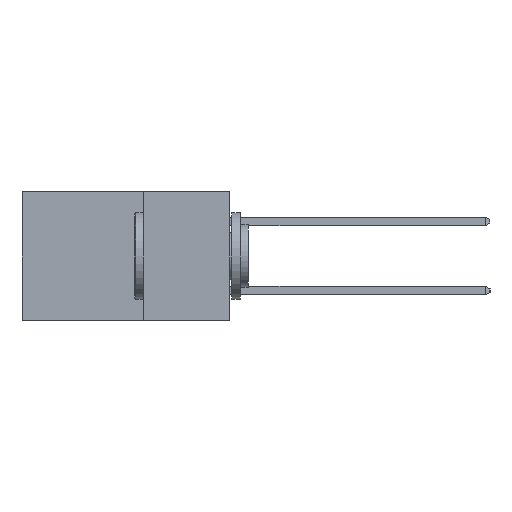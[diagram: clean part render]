
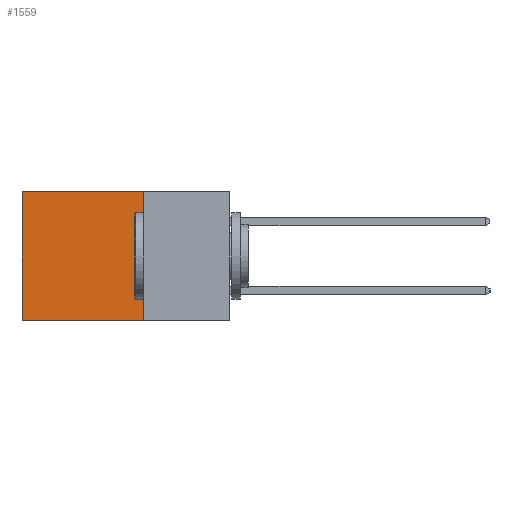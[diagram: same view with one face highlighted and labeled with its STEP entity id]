
A CAD part, left-side view. The second image highlights one B-rep face of the part: STEP entity #1559.
In plain terms, the highlighted planar face has unit normal (-1, 0, 0).
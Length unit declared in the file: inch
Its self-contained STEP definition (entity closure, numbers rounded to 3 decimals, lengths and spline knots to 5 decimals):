
#1008 = AXIS2_PLACEMENT_3D ( 'NONE', #8813, #7997, #16315 ) ;
#1194 = ORIENTED_EDGE ( 'NONE', *, *, #7475, .F. ) ;
#1559 = ADVANCED_FACE ( 'NONE', ( #24263 ), #5330, .F. ) ;
#2029 = CARTESIAN_POINT ( 'NONE',  ( 0.2615, 0.25, -0.37 ) ) ;
#2260 = ORIENTED_EDGE ( 'NONE', *, *, #23071, .T. ) ;
#2371 = VECTOR ( 'NONE', #18679, 39.37008 ) ;
#4174 = DIRECTION ( 'NONE',  ( 0., 0., -1. ) ) ;
#5225 = VERTEX_POINT ( 'NONE', #13977 ) ;
#5330 = PLANE ( 'NONE',  #1008 ) ;
#5928 = EDGE_CURVE ( 'NONE', #17173, #8395, #12949, .T. ) ;
#6491 = ORIENTED_EDGE ( 'NONE', *, *, #5928, .F. ) ;
#7475 = EDGE_CURVE ( 'NONE', #8395, #22567, #9913, .T. ) ;
#7939 = VECTOR ( 'NONE', #23705, 39.37008 ) ;
#7997 = DIRECTION ( 'NONE',  ( 1., 0., 0. ) ) ;
#8395 = VERTEX_POINT ( 'NONE', #2029 ) ;
#8813 = CARTESIAN_POINT ( 'NONE',  ( 0.2615, 0.25, -0.37 ) ) ;
#9248 = CARTESIAN_POINT ( 'NONE',  ( 0.2615, 0.25, 0. ) ) ;
#9913 = LINE ( 'NONE', #11922, #14915 ) ;
#9955 = CARTESIAN_POINT ( 'NONE',  ( 0.2615, 0.6, -0.37 ) ) ;
#11918 = DIRECTION ( 'NONE',  ( 0., 1., 0. ) ) ;
#11922 = CARTESIAN_POINT ( 'NONE',  ( 0.2615, 0.25, -0.37 ) ) ;
#12949 = LINE ( 'NONE', #23739, #7939 ) ;
#13977 = CARTESIAN_POINT ( 'NONE',  ( 0.2615, 0.6, 0. ) ) ;
#14915 = VECTOR ( 'NONE', #11918, 39.37008 ) ;
#15548 = CARTESIAN_POINT ( 'NONE',  ( 0.2615, 0.6, -0.37 ) ) ;
#15950 = EDGE_LOOP ( 'NONE', ( #19637, #1194, #6491, #2260 ) ) ;
#16315 = DIRECTION ( 'NONE',  ( 0., 0., -1. ) ) ;
#17173 = VERTEX_POINT ( 'NONE', #9248 ) ;
#17529 = LINE ( 'NONE', #20540, #2371 ) ;
#18679 = DIRECTION ( 'NONE',  ( 0., 1., 0. ) ) ;
#19273 = LINE ( 'NONE', #15548, #19844 ) ;
#19637 = ORIENTED_EDGE ( 'NONE', *, *, #22540, .T. ) ;
#19844 = VECTOR ( 'NONE', #4174, 39.37008 ) ;
#20540 = CARTESIAN_POINT ( 'NONE',  ( 0.2615, 0.25, 0. ) ) ;
#22540 = EDGE_CURVE ( 'NONE', #5225, #22567, #19273, .T. ) ;
#22567 = VERTEX_POINT ( 'NONE', #9955 ) ;
#23071 = EDGE_CURVE ( 'NONE', #17173, #5225, #17529, .T. ) ;
#23705 = DIRECTION ( 'NONE',  ( 0., 0., -1. ) ) ;
#23739 = CARTESIAN_POINT ( 'NONE',  ( 0.2615, 0.25, -0.37 ) ) ;
#24263 = FACE_OUTER_BOUND ( 'NONE', #15950, .T. ) ;
